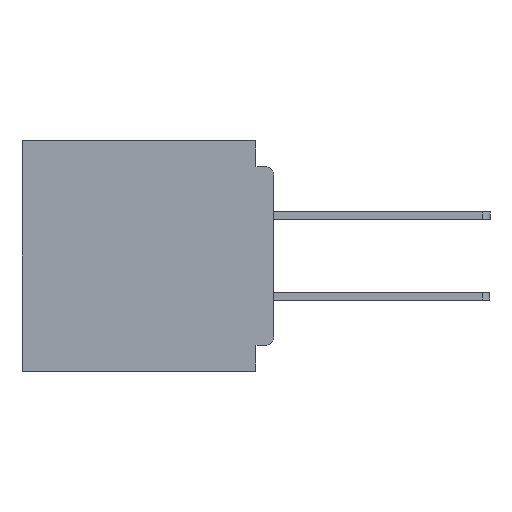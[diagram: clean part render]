
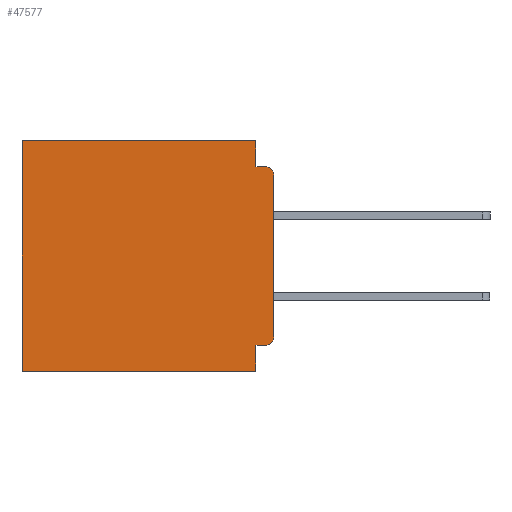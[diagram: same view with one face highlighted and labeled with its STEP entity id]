
A CAD part, left-side view. The second image highlights one B-rep face of the part: STEP entity #47577.
In plain terms, the highlighted planar face has unit normal (-1, 0, 0).
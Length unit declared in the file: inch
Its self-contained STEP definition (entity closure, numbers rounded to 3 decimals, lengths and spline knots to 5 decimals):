
#304 = LINE ( 'NONE', #29310, #47621 ) ;
#862 = CARTESIAN_POINT ( 'NONE',  ( 0.3, 0., -0.06 ) ) ;
#1193 = DIRECTION ( 'NONE',  ( 0., 0., -1. ) ) ;
#1199 = VERTEX_POINT ( 'NONE', #5540 ) ;
#1584 = EDGE_CURVE ( 'NONE', #44558, #1199, #13596, .T. ) ;
#1821 = ORIENTED_EDGE ( 'NONE', *, *, #1584, .F. ) ;
#2300 = CARTESIAN_POINT ( 'NONE',  ( 0.3, 0.015, -0.34 ) ) ;
#2450 = ORIENTED_EDGE ( 'NONE', *, *, #42267, .F. ) ;
#3325 = DIRECTION ( 'NONE',  ( 0., 1., 0. ) ) ;
#3632 = ORIENTED_EDGE ( 'NONE', *, *, #12259, .F. ) ;
#4628 = CARTESIAN_POINT ( 'NONE',  ( 0.3, 0., -0.045 ) ) ;
#5350 = ORIENTED_EDGE ( 'NONE', *, *, #33604, .T. ) ;
#5540 = CARTESIAN_POINT ( 'NONE',  ( 0.3, 0., -0.34 ) ) ;
#6071 = DIRECTION ( 'NONE',  ( 0., 0., -1. ) ) ;
#7161 = ORIENTED_EDGE ( 'NONE', *, *, #41077, .F. ) ;
#7178 = VERTEX_POINT ( 'NONE', #44127 ) ;
#7543 = VECTOR ( 'NONE', #10125, 39.37008 ) ;
#7877 = VERTEX_POINT ( 'NONE', #25915 ) ;
#8808 = CARTESIAN_POINT ( 'NONE',  ( 0.3, 0.437, -0.4 ) ) ;
#9646 = AXIS2_PLACEMENT_3D ( 'NONE', #42444, #20185, #46169 ) ;
#10125 = DIRECTION ( 'NONE',  ( 0., 0., -1. ) ) ;
#10630 = DIRECTION ( 'NONE',  ( 0., 1., 0. ) ) ;
#10767 = VECTOR ( 'NONE', #27119, 39.37008 ) ;
#12233 = AXIS2_PLACEMENT_3D ( 'NONE', #45931, #23751, #1193 ) ;
#12259 = EDGE_CURVE ( 'NONE', #7178, #46969, #26059, .T. ) ;
#12421 = VECTOR ( 'NONE', #34137, 39.37008 ) ;
#13596 = LINE ( 'NONE', #33324, #12421 ) ;
#15284 = DIRECTION ( 'NONE',  ( 0., 1., 0. ) ) ;
#15311 = VERTEX_POINT ( 'NONE', #27900 ) ;
#16086 = VECTOR ( 'NONE', #21959, 39.37008 ) ;
#16160 = PLANE ( 'NONE',  #12233 ) ;
#16562 = ORIENTED_EDGE ( 'NONE', *, *, #19822, .F. ) ;
#17079 = LINE ( 'NONE', #37633, #43263 ) ;
#18076 = EDGE_LOOP ( 'NONE', ( #1821, #5350, #45108, #16562, #37565, #38723, #2450, #3632, #7161, #36990 ) ) ;
#18248 = CARTESIAN_POINT ( 'NONE',  ( 0.3, 0.031, -0.045 ) ) ;
#18394 = DIRECTION ( 'NONE',  ( 0., 0., -1. ) ) ;
#18539 = CARTESIAN_POINT ( 'NONE',  ( 0.3, 0.031, 0. ) ) ;
#19822 = EDGE_CURVE ( 'NONE', #7877, #30620, #21668, .T. ) ;
#20055 = VERTEX_POINT ( 'NONE', #8808 ) ;
#20185 = DIRECTION ( 'NONE',  ( -1., 0., 0. ) ) ;
#20785 = LINE ( 'NONE', #4628, #10767 ) ;
#21142 = EDGE_CURVE ( 'NONE', #30667, #1199, #22729, .T. ) ;
#21229 = CARTESIAN_POINT ( 'NONE',  ( 0.3, 0.437, 0. ) ) ;
#21668 = LINE ( 'NONE', #18539, #40274 ) ;
#21959 = DIRECTION ( 'NONE',  ( 0., 0., -1. ) ) ;
#22729 = CIRCLE ( 'NONE', #23148, 0.015 ) ;
#22730 = EDGE_CURVE ( 'NONE', #30620, #15311, #20785, .T. ) ;
#23148 = AXIS2_PLACEMENT_3D ( 'NONE', #2300, #28548, #6071 ) ;
#23751 = DIRECTION ( 'NONE',  ( 1., 0., 0. ) ) ;
#25395 = CARTESIAN_POINT ( 'NONE',  ( 0.3, 0.031, -0.4 ) ) ;
#25915 = CARTESIAN_POINT ( 'NONE',  ( 0.3, 0.031, 0. ) ) ;
#26059 = LINE ( 'NONE', #25395, #16086 ) ;
#27119 = DIRECTION ( 'NONE',  ( 0., -1., 0. ) ) ;
#27900 = CARTESIAN_POINT ( 'NONE',  ( 0.3, 0.015, -0.045 ) ) ;
#28548 = DIRECTION ( 'NONE',  ( -1., 0., 0. ) ) ;
#29310 = CARTESIAN_POINT ( 'NONE',  ( 0.3, 0., -0.4 ) ) ;
#30620 = VERTEX_POINT ( 'NONE', #18248 ) ;
#30667 = VERTEX_POINT ( 'NONE', #37120 ) ;
#31163 = EDGE_CURVE ( 'NONE', #45419, #20055, #37373, .T. ) ;
#33324 = CARTESIAN_POINT ( 'NONE',  ( 0.3, 0., -0.4 ) ) ;
#33604 = EDGE_CURVE ( 'NONE', #44558, #15311, #42914, .T. ) ;
#34137 = DIRECTION ( 'NONE',  ( 0., 0., -1. ) ) ;
#36044 = VECTOR ( 'NONE', #3325, 39.37008 ) ;
#36543 = LINE ( 'NONE', #48022, #36044 ) ;
#36990 = ORIENTED_EDGE ( 'NONE', *, *, #21142, .T. ) ;
#37120 = CARTESIAN_POINT ( 'NONE',  ( 0.3, 0.015, -0.355 ) ) ;
#37373 = LINE ( 'NONE', #40005, #7543 ) ;
#37565 = ORIENTED_EDGE ( 'NONE', *, *, #45138, .T. ) ;
#37633 = CARTESIAN_POINT ( 'NONE',  ( 0.3, 0., 0. ) ) ;
#38531 = CARTESIAN_POINT ( 'NONE',  ( 0.3, 0.031, -0.4 ) ) ;
#38723 = ORIENTED_EDGE ( 'NONE', *, *, #31163, .T. ) ;
#40005 = CARTESIAN_POINT ( 'NONE',  ( 0.3, 0.437, -0.4 ) ) ;
#40274 = VECTOR ( 'NONE', #18394, 39.37008 ) ;
#41077 = EDGE_CURVE ( 'NONE', #30667, #7178, #36543, .T. ) ;
#41945 = FACE_OUTER_BOUND ( 'NONE', #18076, .T. ) ;
#42267 = EDGE_CURVE ( 'NONE', #46969, #20055, #304, .T. ) ;
#42444 = CARTESIAN_POINT ( 'NONE',  ( 0.3, 0.015, -0.06 ) ) ;
#42914 = CIRCLE ( 'NONE', #9646, 0.015 ) ;
#43263 = VECTOR ( 'NONE', #15284, 39.37008 ) ;
#44127 = CARTESIAN_POINT ( 'NONE',  ( 0.3, 0.031, -0.355 ) ) ;
#44558 = VERTEX_POINT ( 'NONE', #862 ) ;
#45108 = ORIENTED_EDGE ( 'NONE', *, *, #22730, .F. ) ;
#45138 = EDGE_CURVE ( 'NONE', #7877, #45419, #17079, .T. ) ;
#45419 = VERTEX_POINT ( 'NONE', #21229 ) ;
#45931 = CARTESIAN_POINT ( 'NONE',  ( 0.3, 0., -0.4 ) ) ;
#46169 = DIRECTION ( 'NONE',  ( 0., 0., -1. ) ) ;
#46969 = VERTEX_POINT ( 'NONE', #38531 ) ;
#47577 = ADVANCED_FACE ( 'NONE', ( #41945 ), #16160, .F. ) ;
#47621 = VECTOR ( 'NONE', #10630, 39.37008 ) ;
#48022 = CARTESIAN_POINT ( 'NONE',  ( 0.3, 0., -0.355 ) ) ;
